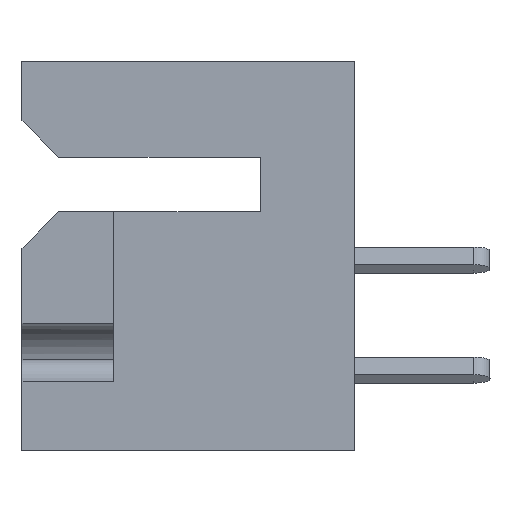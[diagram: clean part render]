
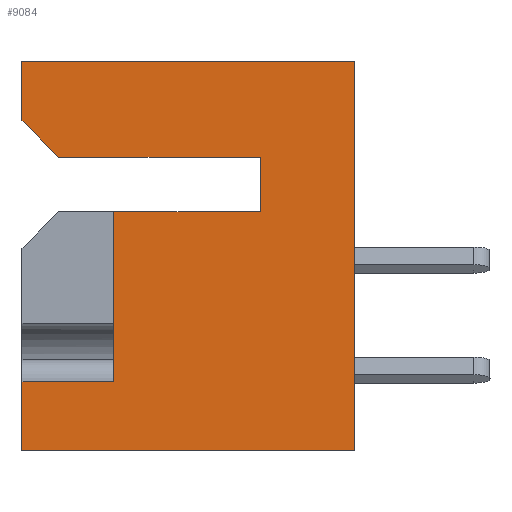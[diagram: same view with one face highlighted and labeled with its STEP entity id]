
A CAD part, left-side view. The second image highlights one B-rep face of the part: STEP entity #9084.
In plain terms, the highlighted planar face has unit normal (-1, 0, 0).
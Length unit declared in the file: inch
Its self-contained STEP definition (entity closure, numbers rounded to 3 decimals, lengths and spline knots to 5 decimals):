
#43 = DIRECTION ( 'NONE',  ( 0., 0., 1. ) ) ;
#161 = LINE ( 'NONE', #10915, #17889 ) ;
#167 = DIRECTION ( 'NONE',  ( 0., -1., 0. ) ) ;
#370 = ORIENTED_EDGE ( 'NONE', *, *, #21115, .F. ) ;
#416 = LINE ( 'NONE', #2150, #10597 ) ;
#920 = LINE ( 'NONE', #15640, #1464 ) ;
#1095 = DIRECTION ( 'NONE',  ( 0., 1., 0. ) ) ;
#1429 = LINE ( 'NONE', #21956, #9979 ) ;
#1464 = VECTOR ( 'NONE', #43, 39.37008 ) ;
#1524 = LINE ( 'NONE', #1720, #20022 ) ;
#1570 = CARTESIAN_POINT ( 'NONE',  ( 0., 0.453, -0.437 ) ) ;
#1720 = CARTESIAN_POINT ( 'NONE',  ( 0., 0.453, 0. ) ) ;
#1819 = VECTOR ( 'NONE', #8195, 39.37008 ) ;
#2149 = LINE ( 'NONE', #18162, #17709 ) ;
#2150 = CARTESIAN_POINT ( 'NONE',  ( 0., 0.128, -0.205 ) ) ;
#2699 = EDGE_CURVE ( 'NONE', #11091, #3152, #920, .T. ) ;
#2736 = ORIENTED_EDGE ( 'NONE', *, *, #10615, .F. ) ;
#3152 = VERTEX_POINT ( 'NONE', #7360 ) ;
#3190 = LINE ( 'NONE', #20374, #13920 ) ;
#3607 = ORIENTED_EDGE ( 'NONE', *, *, #19745, .F. ) ;
#4153 = LINE ( 'NONE', #15388, #16225 ) ;
#5652 = DIRECTION ( 'NONE',  ( 0., 0., -1. ) ) ;
#6114 = AXIS2_PLACEMENT_3D ( 'NONE', #10359, #12084, #5652 ) ;
#6343 = ORIENTED_EDGE ( 'NONE', *, *, #12328, .T. ) ;
#6524 = CARTESIAN_POINT ( 'NONE',  ( 0., 0.128, -0.205 ) ) ;
#7360 = CARTESIAN_POINT ( 'NONE',  ( 0., 0., 0. ) ) ;
#8195 = DIRECTION ( 'NONE',  ( 0., 0., 1. ) ) ;
#8663 = EDGE_CURVE ( 'NONE', #12166, #16602, #9565, .T. ) ;
#8999 = PLANE ( 'NONE',  #6114 ) ;
#9084 = ADVANCED_FACE ( 'NONE', ( #11971 ), #8999, .F. ) ;
#9565 = LINE ( 'NONE', #21977, #1819 ) ;
#9979 = VECTOR ( 'NONE', #20269, 39.37008 ) ;
#10359 = CARTESIAN_POINT ( 'NONE',  ( 0., 0.453, 0. ) ) ;
#10597 = VECTOR ( 'NONE', #12464, 39.37008 ) ;
#10615 = EDGE_CURVE ( 'NONE', #16957, #15385, #3190, .T. ) ;
#10814 = VECTOR ( 'NONE', #11157, 39.37008 ) ;
#10915 = CARTESIAN_POINT ( 'NONE',  ( 0., 0.328, -0.437 ) ) ;
#11091 = VERTEX_POINT ( 'NONE', #17885 ) ;
#11157 = DIRECTION ( 'NONE',  ( 0., 0., 1. ) ) ;
#11656 = CARTESIAN_POINT ( 'NONE',  ( 0., 0.453, -0.081 ) ) ;
#11971 = FACE_OUTER_BOUND ( 'NONE', #16550, .T. ) ;
#12084 = DIRECTION ( 'NONE',  ( 1., 0., 0. ) ) ;
#12166 = VERTEX_POINT ( 'NONE', #13930 ) ;
#12328 = EDGE_CURVE ( 'NONE', #12166, #15385, #161, .T. ) ;
#12464 = DIRECTION ( 'NONE',  ( 0., 1., 0. ) ) ;
#12721 = EDGE_CURVE ( 'NONE', #15317, #16602, #416, .T. ) ;
#12744 = ORIENTED_EDGE ( 'NONE', *, *, #22263, .T. ) ;
#13041 = DIRECTION ( 'NONE',  ( 0., 1., 0. ) ) ;
#13082 = EDGE_CURVE ( 'NONE', #20824, #3152, #4153, .T. ) ;
#13366 = CARTESIAN_POINT ( 'NONE',  ( 0., 0.128, -0.131 ) ) ;
#13371 = DIRECTION ( 'NONE',  ( 0., 0., 1. ) ) ;
#13554 = EDGE_CURVE ( 'NONE', #15317, #19163, #14833, .T. ) ;
#13629 = ORIENTED_EDGE ( 'NONE', *, *, #13082, .F. ) ;
#13920 = VECTOR ( 'NONE', #13371, 39.37008 ) ;
#13930 = CARTESIAN_POINT ( 'NONE',  ( 0., 0.328, -0.437 ) ) ;
#14253 = VERTEX_POINT ( 'NONE', #11656 ) ;
#14303 = CARTESIAN_POINT ( 'NONE',  ( 0., 0.453, -0.531 ) ) ;
#14482 = VERTEX_POINT ( 'NONE', #15854 ) ;
#14670 = CARTESIAN_POINT ( 'NONE',  ( 0., 0.128, -0.131 ) ) ;
#14833 = LINE ( 'NONE', #14670, #10814 ) ;
#15317 = VERTEX_POINT ( 'NONE', #6524 ) ;
#15385 = VERTEX_POINT ( 'NONE', #1570 ) ;
#15388 = CARTESIAN_POINT ( 'NONE',  ( 0., 0.453, 0. ) ) ;
#15640 = CARTESIAN_POINT ( 'NONE',  ( 0., 0., 0. ) ) ;
#15854 = CARTESIAN_POINT ( 'NONE',  ( 0., 0.403, -0.131 ) ) ;
#15946 = VECTOR ( 'NONE', #167, 39.37008 ) ;
#16225 = VECTOR ( 'NONE', #20362, 39.37008 ) ;
#16550 = EDGE_LOOP ( 'NONE', ( #6343, #2736, #12744, #21213, #13629, #370, #22115, #3607, #18584, #17204, #19922 ) ) ;
#16602 = VERTEX_POINT ( 'NONE', #18531 ) ;
#16957 = VERTEX_POINT ( 'NONE', #14303 ) ;
#17167 = DIRECTION ( 'NONE',  ( 0., 0., 1. ) ) ;
#17204 = ORIENTED_EDGE ( 'NONE', *, *, #12721, .T. ) ;
#17709 = VECTOR ( 'NONE', #13041, 39.37008 ) ;
#17880 = EDGE_CURVE ( 'NONE', #14253, #14482, #1429, .T. ) ;
#17885 = CARTESIAN_POINT ( 'NONE',  ( 0., 0., -0.531 ) ) ;
#17889 = VECTOR ( 'NONE', #1095, 39.37008 ) ;
#18162 = CARTESIAN_POINT ( 'NONE',  ( 0., 0.128, -0.131 ) ) ;
#18531 = CARTESIAN_POINT ( 'NONE',  ( 0., 0.328, -0.205 ) ) ;
#18584 = ORIENTED_EDGE ( 'NONE', *, *, #13554, .F. ) ;
#18689 = CARTESIAN_POINT ( 'NONE',  ( 0., 0.453, -0.531 ) ) ;
#18886 = LINE ( 'NONE', #18689, #15946 ) ;
#19163 = VERTEX_POINT ( 'NONE', #13366 ) ;
#19641 = CARTESIAN_POINT ( 'NONE',  ( 0., 0.453, 0. ) ) ;
#19745 = EDGE_CURVE ( 'NONE', #19163, #14482, #2149, .T. ) ;
#19922 = ORIENTED_EDGE ( 'NONE', *, *, #8663, .F. ) ;
#20022 = VECTOR ( 'NONE', #17167, 39.37008 ) ;
#20269 = DIRECTION ( 'NONE',  ( 0., -0.707, -0.707 ) ) ;
#20362 = DIRECTION ( 'NONE',  ( 0., -1., 0. ) ) ;
#20374 = CARTESIAN_POINT ( 'NONE',  ( 0., 0.453, 0. ) ) ;
#20824 = VERTEX_POINT ( 'NONE', #19641 ) ;
#21115 = EDGE_CURVE ( 'NONE', #14253, #20824, #1524, .T. ) ;
#21213 = ORIENTED_EDGE ( 'NONE', *, *, #2699, .T. ) ;
#21956 = CARTESIAN_POINT ( 'NONE',  ( 0., 0.403, -0.131 ) ) ;
#21977 = CARTESIAN_POINT ( 'NONE',  ( 0., 0.328, -0.205 ) ) ;
#22115 = ORIENTED_EDGE ( 'NONE', *, *, #17880, .T. ) ;
#22263 = EDGE_CURVE ( 'NONE', #16957, #11091, #18886, .T. ) ;
